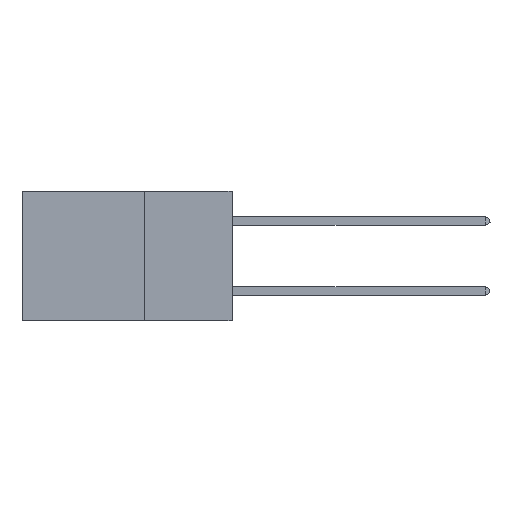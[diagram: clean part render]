
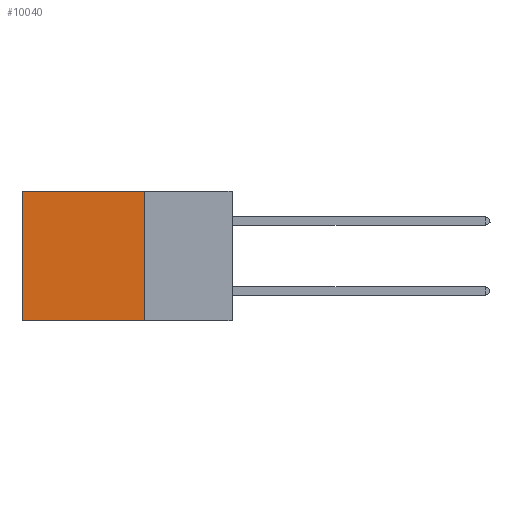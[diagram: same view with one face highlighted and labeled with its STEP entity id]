
A CAD part, left-side view. The second image highlights one B-rep face of the part: STEP entity #10040.
In plain terms, the highlighted planar face has unit normal (-1, 0, 0).
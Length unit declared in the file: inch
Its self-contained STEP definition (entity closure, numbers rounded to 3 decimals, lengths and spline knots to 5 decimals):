
#216 = EDGE_LOOP ( 'NONE', ( #9707, #14095, #8110, #3525 ) ) ;
#424 = FACE_OUTER_BOUND ( 'NONE', #216, .T. ) ;
#527 = EDGE_CURVE ( 'NONE', #8597, #18973, #2638, .T. ) ;
#1082 = AXIS2_PLACEMENT_3D ( 'NONE', #16668, #7890, #18079 ) ;
#1447 = CARTESIAN_POINT ( 'NONE',  ( 0.2875, 0.25, 0. ) ) ;
#1537 = VECTOR ( 'NONE', #6597, 39.37008 ) ;
#1737 = VERTEX_POINT ( 'NONE', #5357 ) ;
#1805 = CARTESIAN_POINT ( 'NONE',  ( 0.2875, 0.6, -0.37 ) ) ;
#2638 = LINE ( 'NONE', #13787, #17785 ) ;
#3525 = ORIENTED_EDGE ( 'NONE', *, *, #527, .T. ) ;
#4037 = VECTOR ( 'NONE', #18477, 39.37008 ) ;
#5149 = LINE ( 'NONE', #16827, #1537 ) ;
#5357 = CARTESIAN_POINT ( 'NONE',  ( 0.2875, 0.25, -0.37 ) ) ;
#6436 = PLANE ( 'NONE',  #1082 ) ;
#6597 = DIRECTION ( 'NONE',  ( 0., 1., 0. ) ) ;
#7890 = DIRECTION ( 'NONE',  ( 1., 0., 0. ) ) ;
#7937 = LINE ( 'NONE', #9795, #4037 ) ;
#8110 = ORIENTED_EDGE ( 'NONE', *, *, #17015, .F. ) ;
#8597 = VERTEX_POINT ( 'NONE', #11854 ) ;
#9707 = ORIENTED_EDGE ( 'NONE', *, *, #10952, .T. ) ;
#9795 = CARTESIAN_POINT ( 'NONE',  ( 0.2875, 0.6, 0. ) ) ;
#10040 = ADVANCED_FACE ( 'NONE', ( #424 ), #6436, .F. ) ;
#10876 = LINE ( 'NONE', #1447, #18128 ) ;
#10952 = EDGE_CURVE ( 'NONE', #18973, #14137, #7937, .T. ) ;
#11854 = CARTESIAN_POINT ( 'NONE',  ( 0.2875, 0.25, 0. ) ) ;
#13327 = EDGE_CURVE ( 'NONE', #1737, #14137, #5149, .T. ) ;
#13787 = CARTESIAN_POINT ( 'NONE',  ( 0.2875, 0.25, 0. ) ) ;
#14095 = ORIENTED_EDGE ( 'NONE', *, *, #13327, .F. ) ;
#14137 = VERTEX_POINT ( 'NONE', #1805 ) ;
#14798 = DIRECTION ( 'NONE',  ( 0., 0., -1. ) ) ;
#14925 = CARTESIAN_POINT ( 'NONE',  ( 0.2875, 0.6, 0. ) ) ;
#14946 = DIRECTION ( 'NONE',  ( 0., 1., 0. ) ) ;
#16668 = CARTESIAN_POINT ( 'NONE',  ( 0.2875, 0.25, 0. ) ) ;
#16827 = CARTESIAN_POINT ( 'NONE',  ( 0.2875, 0.25, -0.37 ) ) ;
#17015 = EDGE_CURVE ( 'NONE', #8597, #1737, #10876, .T. ) ;
#17785 = VECTOR ( 'NONE', #14946, 39.37008 ) ;
#18079 = DIRECTION ( 'NONE',  ( 0., 0., -1. ) ) ;
#18128 = VECTOR ( 'NONE', #14798, 39.37008 ) ;
#18477 = DIRECTION ( 'NONE',  ( 0., 0., -1. ) ) ;
#18973 = VERTEX_POINT ( 'NONE', #14925 ) ;
